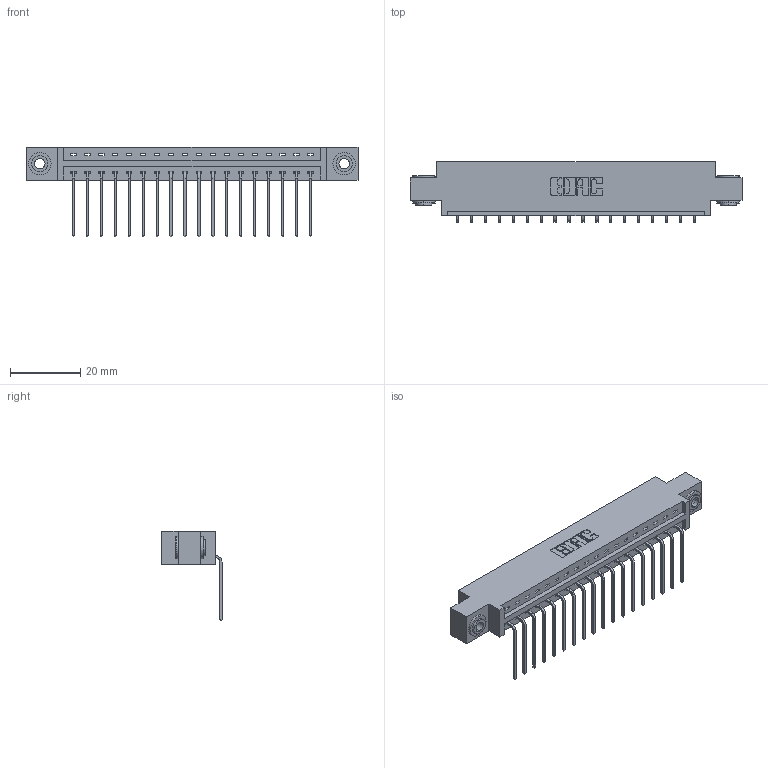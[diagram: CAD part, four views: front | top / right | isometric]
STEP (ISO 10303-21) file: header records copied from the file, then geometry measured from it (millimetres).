
FILE_DESCRIPTION (( 'STEP AP203' ), '1' );
FILE_NAME ('337-018-559-603.STEP', '2019-09-28T20:41:47', ( '' ), ( '' ), 'SwSTEP 2.0', 'SolidWorks 2016', '' );
FILE_SCHEMA (( 'CONFIG_CONTROL_DESIGN' ));
Length unit declared in the file: inch
Products named in the file (4): 345-250-002_345-250-002-102; 337 Part_0.170 Offset - 0.156 Dia-TH; 345-292-001_558 559 Tail - 1; 337-018-559-603
Assembly tree (21 placements, depth 2):
  337-018-559-603
    337 Part_0.170 Offset - 0.156 Dia-TH
    345-292-001_558 559 Tail - 1  x18
    345-250-002_345-250-002-102  x2
Bounding box: 94.34 x 17.09 x 25.53 mm (x, y, z)
Volume: 9466.1 mm3; surface area: 10346.2 mm2
Topology: 21 solids, 21 shells, 1308 faces, 3891 edges, 2566 vertices
Faces by surface type: plane 948, cylinder 352, cone 8
Entity records: 17350 total; most frequent: CARTESIAN_POINT 2999, ORIENTED_EDGE 2946, DIRECTION 2607, EDGE_CURVE 1473, LINE 1321, VECTOR 1321, VERTEX_POINT 978, AXIS2_PLACEMENT_3D 643
